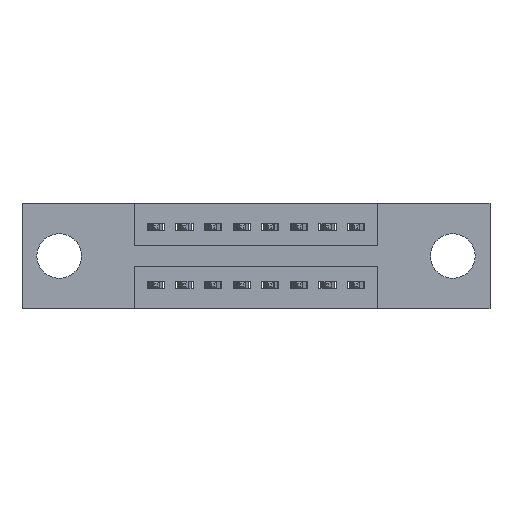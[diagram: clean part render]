
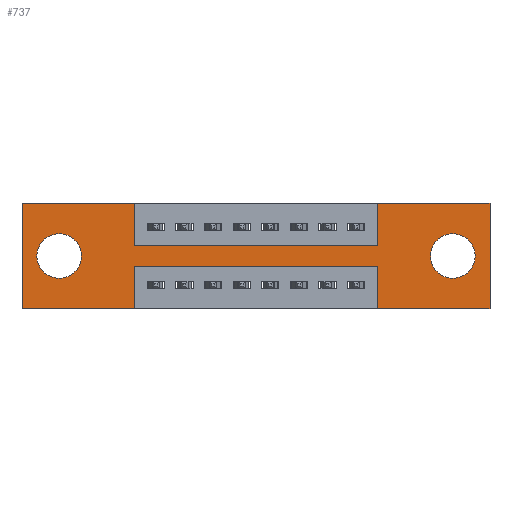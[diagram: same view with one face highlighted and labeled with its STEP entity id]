
A CAD part, front view. The second image highlights one B-rep face of the part: STEP entity #737.
In plain terms, the highlighted planar face has unit normal (0, -1, 0).
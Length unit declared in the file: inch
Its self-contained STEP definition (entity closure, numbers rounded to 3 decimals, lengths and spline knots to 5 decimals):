
#107 = CIRCLE ( 'NONE', #9408, 0.078 ) ;
#205 = DIRECTION ( 'NONE',  ( -1., 0., 0. ) ) ;
#224 = EDGE_CURVE ( 'NONE', #1174, #9063, #10647, .T. ) ;
#230 = ORIENTED_EDGE ( 'NONE', *, *, #6662, .F. ) ;
#238 = EDGE_CURVE ( 'NONE', #6436, #1425, #10566, .T. ) ;
#247 = CARTESIAN_POINT ( 'NONE',  ( 0., 0., 0. ) ) ;
#252 = VECTOR ( 'NONE', #7357, 39.37008 ) ;
#293 = CARTESIAN_POINT ( 'NONE',  ( 1.505, 0., -0.185 ) ) ;
#325 = ORIENTED_EDGE ( 'NONE', *, *, #10214, .T. ) ;
#528 = ORIENTED_EDGE ( 'NONE', *, *, #1143, .F. ) ;
#651 = EDGE_CURVE ( 'NONE', #4838, #9377, #10641, .T. ) ;
#716 = CARTESIAN_POINT ( 'NONE',  ( 0., 0., -0.37 ) ) ;
#737 = ADVANCED_FACE ( 'NONE', ( #7977, #3615, #9721 ), #7113, .T. ) ;
#863 = ORIENTED_EDGE ( 'NONE', *, *, #10335, .F. ) ;
#879 = DIRECTION ( 'NONE',  ( 1., 0., 0. ) ) ;
#1143 = EDGE_CURVE ( 'NONE', #10810, #3254, #10488, .T. ) ;
#1174 = VERTEX_POINT ( 'NONE', #1912 ) ;
#1319 = LINE ( 'NONE', #8382, #2386 ) ;
#1425 = VERTEX_POINT ( 'NONE', #10538 ) ;
#1627 = CARTESIAN_POINT ( 'NONE',  ( 1.635, 0., 0. ) ) ;
#1698 = DIRECTION ( 'NONE',  ( 0., 1., 0. ) ) ;
#1912 = CARTESIAN_POINT ( 'NONE',  ( 0., 0., -0.37 ) ) ;
#1913 = CARTESIAN_POINT ( 'NONE',  ( 0.3925, 0., -0.22 ) ) ;
#1914 = LINE ( 'NONE', #2606, #7522 ) ;
#1936 = LINE ( 'NONE', #8066, #6518 ) ;
#2203 = ORIENTED_EDGE ( 'NONE', *, *, #8274, .F. ) ;
#2272 = VECTOR ( 'NONE', #11243, 39.37008 ) ;
#2298 = VECTOR ( 'NONE', #3334, 39.37008 ) ;
#2386 = VECTOR ( 'NONE', #879, 39.37008 ) ;
#2500 = VERTEX_POINT ( 'NONE', #9143 ) ;
#2561 = CARTESIAN_POINT ( 'NONE',  ( 0.3925, 0., -0.37 ) ) ;
#2606 = CARTESIAN_POINT ( 'NONE',  ( 0.3925, 0., -0.22 ) ) ;
#2899 = LINE ( 'NONE', #5836, #4647 ) ;
#2908 = ORIENTED_EDGE ( 'NONE', *, *, #8258, .F. ) ;
#2975 = VERTEX_POINT ( 'NONE', #9352 ) ;
#3119 = DIRECTION ( 'NONE',  ( -1., 0., 0. ) ) ;
#3170 = CARTESIAN_POINT ( 'NONE',  ( 1.2425, 0., -0.15 ) ) ;
#3172 = VECTOR ( 'NONE', #3119, 39.37008 ) ;
#3254 = VERTEX_POINT ( 'NONE', #10565 ) ;
#3334 = DIRECTION ( 'NONE',  ( 0., 0., -1. ) ) ;
#3405 = CIRCLE ( 'NONE', #6340, 0.078 ) ;
#3499 = CARTESIAN_POINT ( 'NONE',  ( 0.13, 0., -0.107 ) ) ;
#3615 = FACE_BOUND ( 'NONE', #5124, .T. ) ;
#3732 = DIRECTION ( 'NONE',  ( 0., 0., 1. ) ) ;
#3746 = VERTEX_POINT ( 'NONE', #1913 ) ;
#3769 = ORIENTED_EDGE ( 'NONE', *, *, #11067, .F. ) ;
#3946 = EDGE_CURVE ( 'NONE', #1425, #4838, #1319, .T. ) ;
#4094 = VECTOR ( 'NONE', #9785, 39.37008 ) ;
#4278 = LINE ( 'NONE', #716, #2272 ) ;
#4358 = AXIS2_PLACEMENT_3D ( 'NONE', #7452, #6637, #5801 ) ;
#4647 = VECTOR ( 'NONE', #9305, 39.37008 ) ;
#4701 = CARTESIAN_POINT ( 'NONE',  ( 1.635, 0., 0. ) ) ;
#4742 = LINE ( 'NONE', #7617, #6666 ) ;
#4762 = ORIENTED_EDGE ( 'NONE', *, *, #651, .F. ) ;
#4838 = VERTEX_POINT ( 'NONE', #1627 ) ;
#4951 = EDGE_LOOP ( 'NONE', ( #9521, #4995 ) ) ;
#4995 = ORIENTED_EDGE ( 'NONE', *, *, #7171, .T. ) ;
#5124 = EDGE_LOOP ( 'NONE', ( #7368, #325 ) ) ;
#5525 = ORIENTED_EDGE ( 'NONE', *, *, #3946, .F. ) ;
#5801 = DIRECTION ( 'NONE',  ( 0., 0., 1. ) ) ;
#5836 = CARTESIAN_POINT ( 'NONE',  ( 0., 0., 0. ) ) ;
#5850 = EDGE_LOOP ( 'NONE', ( #3769, #863, #9490, #2908, #4762, #5525, #8855, #7981, #528, #2203, #10718, #230 ) ) ;
#5893 = DIRECTION ( 'NONE',  ( 0., 0., -1. ) ) ;
#5950 = VERTEX_POINT ( 'NONE', #9831 ) ;
#5989 = EDGE_CURVE ( 'NONE', #3254, #6436, #4742, .T. ) ;
#6074 = DIRECTION ( 'NONE',  ( 0., 0., -1. ) ) ;
#6253 = DIRECTION ( 'NONE',  ( 0., -1., 0. ) ) ;
#6340 = AXIS2_PLACEMENT_3D ( 'NONE', #10389, #1698, #5893 ) ;
#6436 = VERTEX_POINT ( 'NONE', #3170 ) ;
#6518 = VECTOR ( 'NONE', #10573, 39.37008 ) ;
#6548 = VERTEX_POINT ( 'NONE', #7710 ) ;
#6637 = DIRECTION ( 'NONE',  ( 0., 1., 0. ) ) ;
#6662 = EDGE_CURVE ( 'NONE', #8894, #1174, #4278, .T. ) ;
#6666 = VECTOR ( 'NONE', #7443, 39.37008 ) ;
#6785 = CARTESIAN_POINT ( 'NONE',  ( 0.13, 0., -0.185 ) ) ;
#6961 = VERTEX_POINT ( 'NONE', #9447 ) ;
#7068 = CARTESIAN_POINT ( 'NONE',  ( 0.3925, 0., -0.37 ) ) ;
#7075 = VERTEX_POINT ( 'NONE', #3499 ) ;
#7113 = PLANE ( 'NONE',  #8321 ) ;
#7163 = DIRECTION ( 'NONE',  ( 0., 0., -1. ) ) ;
#7171 = EDGE_CURVE ( 'NONE', #2500, #2975, #107, .T. ) ;
#7357 = DIRECTION ( 'NONE',  ( 0., 0., 1. ) ) ;
#7368 = ORIENTED_EDGE ( 'NONE', *, *, #9076, .T. ) ;
#7443 = DIRECTION ( 'NONE',  ( 1., 0., 0. ) ) ;
#7452 = CARTESIAN_POINT ( 'NONE',  ( 0.13, 0., -0.185 ) ) ;
#7490 = LINE ( 'NONE', #10961, #3172 ) ;
#7522 = VECTOR ( 'NONE', #205, 39.37008 ) ;
#7617 = CARTESIAN_POINT ( 'NONE',  ( 0.3925, 0., -0.15 ) ) ;
#7710 = CARTESIAN_POINT ( 'NONE',  ( 1.2425, 0., -0.22 ) ) ;
#7971 = EDGE_CURVE ( 'NONE', #5950, #6548, #1936, .T. ) ;
#7977 = FACE_BOUND ( 'NONE', #4951, .T. ) ;
#7981 = ORIENTED_EDGE ( 'NONE', *, *, #5989, .F. ) ;
#8066 = CARTESIAN_POINT ( 'NONE',  ( 1.2425, 0., -0.37 ) ) ;
#8258 = EDGE_CURVE ( 'NONE', #9377, #5950, #7490, .T. ) ;
#8274 = EDGE_CURVE ( 'NONE', #9063, #10810, #2899, .T. ) ;
#8321 = AXIS2_PLACEMENT_3D ( 'NONE', #10578, #6253, #7163 ) ;
#8382 = CARTESIAN_POINT ( 'NONE',  ( 0., 0., 0. ) ) ;
#8825 = CARTESIAN_POINT ( 'NONE',  ( 1.635, 0., -0.37 ) ) ;
#8847 = VECTOR ( 'NONE', #3732, 39.37008 ) ;
#8855 = ORIENTED_EDGE ( 'NONE', *, *, #238, .F. ) ;
#8894 = VERTEX_POINT ( 'NONE', #7068 ) ;
#9032 = DIRECTION ( 'NONE',  ( 0., 1., 0. ) ) ;
#9063 = VERTEX_POINT ( 'NONE', #10000 ) ;
#9076 = EDGE_CURVE ( 'NONE', #7075, #6961, #10717, .T. ) ;
#9143 = CARTESIAN_POINT ( 'NONE',  ( 1.505, 0., -0.263 ) ) ;
#9300 = DIRECTION ( 'NONE',  ( 0., 1., 0. ) ) ;
#9305 = DIRECTION ( 'NONE',  ( 1., 0., 0. ) ) ;
#9352 = CARTESIAN_POINT ( 'NONE',  ( 1.505, 0., -0.107 ) ) ;
#9377 = VERTEX_POINT ( 'NONE', #8825 ) ;
#9408 = AXIS2_PLACEMENT_3D ( 'NONE', #293, #9032, #10746 ) ;
#9447 = CARTESIAN_POINT ( 'NONE',  ( 0.13, 0., -0.263 ) ) ;
#9490 = ORIENTED_EDGE ( 'NONE', *, *, #7971, .F. ) ;
#9521 = ORIENTED_EDGE ( 'NONE', *, *, #9679, .T. ) ;
#9679 = EDGE_CURVE ( 'NONE', #2975, #2500, #3405, .T. ) ;
#9721 = FACE_OUTER_BOUND ( 'NONE', #5850, .T. ) ;
#9785 = DIRECTION ( 'NONE',  ( 0., 0., -1. ) ) ;
#9831 = CARTESIAN_POINT ( 'NONE',  ( 1.2425, 0., -0.37 ) ) ;
#9939 = CARTESIAN_POINT ( 'NONE',  ( 0.3925, 0., 0. ) ) ;
#10000 = CARTESIAN_POINT ( 'NONE',  ( 0., 0., 0. ) ) ;
#10214 = EDGE_CURVE ( 'NONE', #6961, #7075, #10432, .T. ) ;
#10242 = AXIS2_PLACEMENT_3D ( 'NONE', #6785, #9300, #10258 ) ;
#10252 = VECTOR ( 'NONE', #6074, 39.37008 ) ;
#10258 = DIRECTION ( 'NONE',  ( 0., 0., 1. ) ) ;
#10335 = EDGE_CURVE ( 'NONE', #6548, #3746, #1914, .T. ) ;
#10389 = CARTESIAN_POINT ( 'NONE',  ( 1.505, 0., -0.185 ) ) ;
#10432 = CIRCLE ( 'NONE', #10242, 0.078 ) ;
#10454 = CARTESIAN_POINT ( 'NONE',  ( 1.2425, 0., 0. ) ) ;
#10488 = LINE ( 'NONE', #10549, #2298 ) ;
#10538 = CARTESIAN_POINT ( 'NONE',  ( 1.2425, 0., 0. ) ) ;
#10549 = CARTESIAN_POINT ( 'NONE',  ( 0.3925, 0., 0. ) ) ;
#10565 = CARTESIAN_POINT ( 'NONE',  ( 0.3925, 0., -0.15 ) ) ;
#10566 = LINE ( 'NONE', #10454, #252 ) ;
#10573 = DIRECTION ( 'NONE',  ( 0., 0., 1. ) ) ;
#10578 = CARTESIAN_POINT ( 'NONE',  ( 0., 0., -0.37 ) ) ;
#10641 = LINE ( 'NONE', #4701, #4094 ) ;
#10647 = LINE ( 'NONE', #247, #8847 ) ;
#10717 = CIRCLE ( 'NONE', #4358, 0.078 ) ;
#10718 = ORIENTED_EDGE ( 'NONE', *, *, #224, .F. ) ;
#10746 = DIRECTION ( 'NONE',  ( 0., 0., -1. ) ) ;
#10810 = VERTEX_POINT ( 'NONE', #9939 ) ;
#10961 = CARTESIAN_POINT ( 'NONE',  ( 0., 0., -0.37 ) ) ;
#11067 = EDGE_CURVE ( 'NONE', #3746, #8894, #11084, .T. ) ;
#11084 = LINE ( 'NONE', #2561, #10252 ) ;
#11243 = DIRECTION ( 'NONE',  ( -1., 0., 0. ) ) ;
